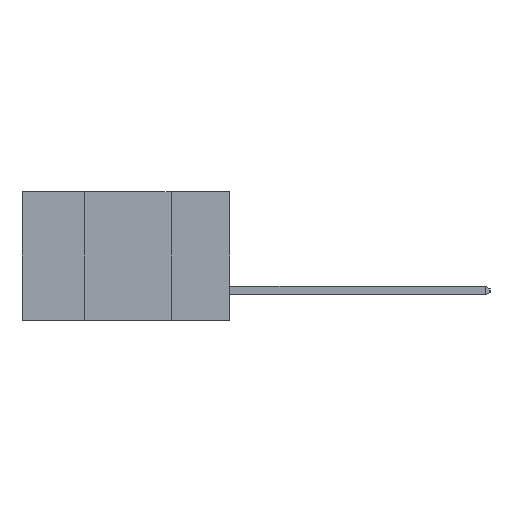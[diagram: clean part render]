
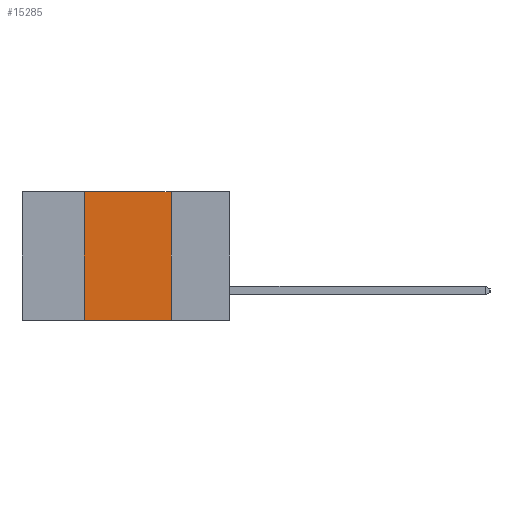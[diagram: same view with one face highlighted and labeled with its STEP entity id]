
A CAD part, left-side view. The second image highlights one B-rep face of the part: STEP entity #15285.
In plain terms, the highlighted planar face has unit normal (-1, 0, 0).
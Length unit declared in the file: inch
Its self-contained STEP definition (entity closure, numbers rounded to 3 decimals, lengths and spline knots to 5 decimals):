
#816 = CARTESIAN_POINT ( 'NONE',  ( 0., 0.17, 0. ) ) ;
#827 = ORIENTED_EDGE ( 'NONE', *, *, #15484, .F. ) ;
#896 = VERTEX_POINT ( 'NONE', #14308 ) ;
#1748 = VECTOR ( 'NONE', #2097, 39.37008 ) ;
#2097 = DIRECTION ( 'NONE',  ( 0., 0., -1. ) ) ;
#3258 = ORIENTED_EDGE ( 'NONE', *, *, #8384, .T. ) ;
#4094 = PLANE ( 'NONE',  #13353 ) ;
#5364 = CARTESIAN_POINT ( 'NONE',  ( 0., 0.42, 0. ) ) ;
#5384 = DIRECTION ( 'NONE',  ( 1., 0., 0. ) ) ;
#5419 = CARTESIAN_POINT ( 'NONE',  ( 0., 0.17, -0.37 ) ) ;
#5722 = DIRECTION ( 'NONE',  ( 0., -1., 0. ) ) ;
#5975 = EDGE_LOOP ( 'NONE', ( #827, #10684, #9465, #3258 ) ) ;
#6433 = EDGE_CURVE ( 'NONE', #11432, #896, #12485, .T. ) ;
#6491 = LINE ( 'NONE', #5364, #12581 ) ;
#8384 = EDGE_CURVE ( 'NONE', #12071, #14029, #12232, .T. ) ;
#8893 = CARTESIAN_POINT ( 'NONE',  ( 0., 0.42, 0. ) ) ;
#9029 = VECTOR ( 'NONE', #15395, 39.37008 ) ;
#9465 = ORIENTED_EDGE ( 'NONE', *, *, #13971, .F. ) ;
#9737 = CARTESIAN_POINT ( 'NONE',  ( 0., 0.6, 0. ) ) ;
#10684 = ORIENTED_EDGE ( 'NONE', *, *, #6433, .F. ) ;
#11432 = VERTEX_POINT ( 'NONE', #8893 ) ;
#11504 = CARTESIAN_POINT ( 'NONE',  ( 0., 0.6, 0. ) ) ;
#12071 = VERTEX_POINT ( 'NONE', #12511 ) ;
#12232 = LINE ( 'NONE', #13102, #9029 ) ;
#12485 = LINE ( 'NONE', #9737, #14109 ) ;
#12511 = CARTESIAN_POINT ( 'NONE',  ( 0., 0.42, -0.37 ) ) ;
#12581 = VECTOR ( 'NONE', #14967, 39.37008 ) ;
#13102 = CARTESIAN_POINT ( 'NONE',  ( 0., 0.6, -0.37 ) ) ;
#13353 = AXIS2_PLACEMENT_3D ( 'NONE', #11504, #5384, #13839 ) ;
#13839 = DIRECTION ( 'NONE',  ( 0., 0., -1. ) ) ;
#13971 = EDGE_CURVE ( 'NONE', #12071, #11432, #6491, .T. ) ;
#14029 = VERTEX_POINT ( 'NONE', #5419 ) ;
#14109 = VECTOR ( 'NONE', #5722, 39.37008 ) ;
#14308 = CARTESIAN_POINT ( 'NONE',  ( 0., 0.17, 0. ) ) ;
#14511 = FACE_OUTER_BOUND ( 'NONE', #5975, .T. ) ;
#14686 = LINE ( 'NONE', #816, #1748 ) ;
#14967 = DIRECTION ( 'NONE',  ( 0., 0., 1. ) ) ;
#15285 = ADVANCED_FACE ( 'NONE', ( #14511 ), #4094, .F. ) ;
#15395 = DIRECTION ( 'NONE',  ( 0., -1., 0. ) ) ;
#15484 = EDGE_CURVE ( 'NONE', #896, #14029, #14686, .T. ) ;
